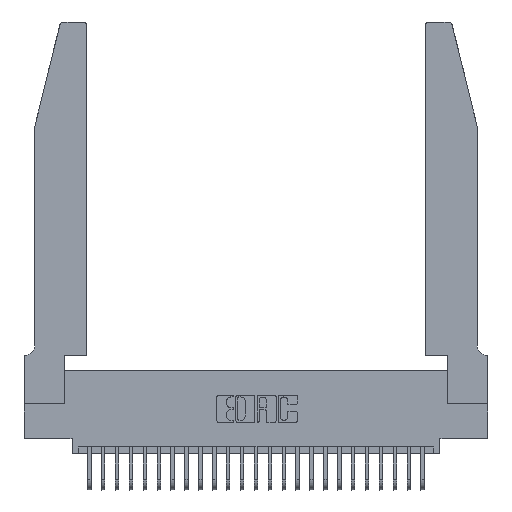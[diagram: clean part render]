
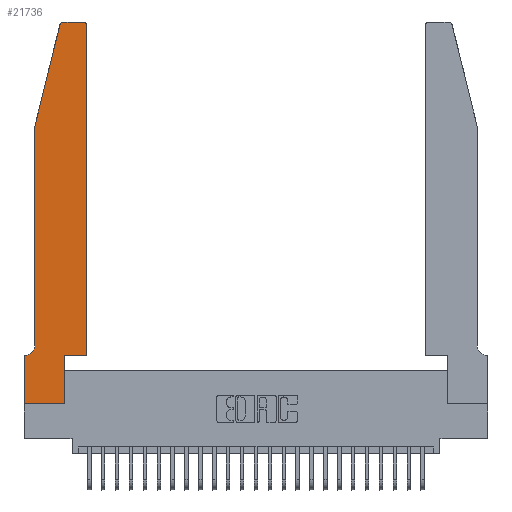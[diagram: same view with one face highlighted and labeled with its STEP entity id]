
A CAD part, top view. The second image highlights one B-rep face of the part: STEP entity #21736.
In plain terms, the highlighted planar face has unit normal (0, 0, 1).
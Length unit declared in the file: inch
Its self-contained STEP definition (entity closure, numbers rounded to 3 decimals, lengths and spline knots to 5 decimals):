
#370 = DIRECTION ( 'NONE',  ( -0.239, -0.971, 0. ) ) ;
#458 = LINE ( 'NONE', #26367, #18158 ) ;
#739 = CARTESIAN_POINT ( 'NONE',  ( 0.0755, 2., 0.37 ) ) ;
#792 = VERTEX_POINT ( 'NONE', #2043 ) ;
#999 = DIRECTION ( 'NONE',  ( 1., 0., 0. ) ) ;
#1038 = EDGE_CURVE ( 'NONE', #14653, #17005, #2026, .T. ) ;
#2026 = LINE ( 'NONE', #13198, #24736 ) ;
#2043 = CARTESIAN_POINT ( 'NONE',  ( 0.25487, 2.72718, 0.37 ) ) ;
#2344 = LINE ( 'NONE', #26648, #13473 ) ;
#2377 = CIRCLE ( 'NONE', #4136, 0.03 ) ;
#2674 = CARTESIAN_POINT ( 'NONE',  ( 0.4205, 2.72, 0.37 ) ) ;
#3915 = CARTESIAN_POINT ( 'NONE',  ( 0.0055, 0.42, 0.37 ) ) ;
#3991 = DIRECTION ( 'NONE',  ( 1., 0., 0. ) ) ;
#4113 = VECTOR ( 'NONE', #16092, 39.37008 ) ;
#4121 = VERTEX_POINT ( 'NONE', #28270 ) ;
#4136 = AXIS2_PLACEMENT_3D ( 'NONE', #2674, #18172, #4959 ) ;
#4201 = LINE ( 'NONE', #13701, #16003 ) ;
#4290 = CARTESIAN_POINT ( 'NONE',  ( 0.284, 2.72, 0.37 ) ) ;
#4513 = LINE ( 'NONE', #6913, #21312 ) ;
#4536 = VERTEX_POINT ( 'NONE', #14696 ) ;
#4736 = EDGE_CURVE ( 'NONE', #6855, #4121, #458, .T. ) ;
#4761 = ORIENTED_EDGE ( 'NONE', *, *, #24069, .T. ) ;
#4855 = ORIENTED_EDGE ( 'NONE', *, *, #20783, .T. ) ;
#4959 = DIRECTION ( 'NONE',  ( 1., 0., 0. ) ) ;
#5266 = LINE ( 'NONE', #25333, #16341 ) ;
#5336 = VERTEX_POINT ( 'NONE', #19955 ) ;
#5622 = VECTOR ( 'NONE', #11057, 39.37008 ) ;
#5817 = CARTESIAN_POINT ( 'NONE',  ( 0.2865, 0., 0.37 ) ) ;
#6170 = DIRECTION ( 'NONE',  ( -1., 0., 0. ) ) ;
#6537 = DIRECTION ( 'NONE',  ( 1., 0., 0. ) ) ;
#6746 = VERTEX_POINT ( 'NONE', #7605 ) ;
#6763 = VERTEX_POINT ( 'NONE', #16480 ) ;
#6855 = VERTEX_POINT ( 'NONE', #21061 ) ;
#6913 = CARTESIAN_POINT ( 'NONE',  ( 0.4505, 0.35, 0.37 ) ) ;
#6969 = DIRECTION ( 'NONE',  ( 0., 1., 0. ) ) ;
#7067 = CARTESIAN_POINT ( 'NONE',  ( 0.4205, 2.75, 0.37 ) ) ;
#7605 = CARTESIAN_POINT ( 'NONE',  ( 0.4505, 2.72, 0.37 ) ) ;
#7697 = CARTESIAN_POINT ( 'NONE',  ( 0., 0.35, 0.37 ) ) ;
#7717 = VERTEX_POINT ( 'NONE', #7067 ) ;
#7966 = LINE ( 'NONE', #26857, #4113 ) ;
#8982 = EDGE_CURVE ( 'NONE', #6763, #792, #11916, .T. ) ;
#9638 = EDGE_CURVE ( 'NONE', #7717, #6763, #17377, .T. ) ;
#10096 = EDGE_CURVE ( 'NONE', #22844, #6855, #12187, .T. ) ;
#10583 = ORIENTED_EDGE ( 'NONE', *, *, #1038, .T. ) ;
#10942 = EDGE_CURVE ( 'NONE', #5336, #6746, #4513, .T. ) ;
#11019 = EDGE_CURVE ( 'NONE', #6746, #7717, #2377, .T. ) ;
#11057 = DIRECTION ( 'NONE',  ( -1., 0., 0. ) ) ;
#11712 = EDGE_CURVE ( 'NONE', #4536, #5336, #7966, .T. ) ;
#11761 = AXIS2_PLACEMENT_3D ( 'NONE', #3915, #19330, #6170 ) ;
#11916 = CIRCLE ( 'NONE', #24123, 0.03 ) ;
#12187 = CIRCLE ( 'NONE', #11761, 0.07 ) ;
#12726 = CARTESIAN_POINT ( 'NONE',  ( 0.0755, 0.42, 0.37 ) ) ;
#13100 = CARTESIAN_POINT ( 'NONE',  ( 0., 0., 0.37 ) ) ;
#13198 = CARTESIAN_POINT ( 'NONE',  ( 0., 0., 0.37 ) ) ;
#13473 = VECTOR ( 'NONE', #6969, 39.37008 ) ;
#13474 = DIRECTION ( 'NONE',  ( 0., 1., 0. ) ) ;
#13701 = CARTESIAN_POINT ( 'NONE',  ( 0.0755, 2., 0.37 ) ) ;
#14337 = DIRECTION ( 'NONE',  ( 0., 0., 1. ) ) ;
#14653 = VERTEX_POINT ( 'NONE', #13100 ) ;
#14696 = CARTESIAN_POINT ( 'NONE',  ( 0.2865, 0.35, 0.37 ) ) ;
#14773 = ORIENTED_EDGE ( 'NONE', *, *, #10942, .T. ) ;
#15584 = DIRECTION ( 'NONE',  ( -1., 0., 0. ) ) ;
#16003 = VECTOR ( 'NONE', #370, 39.37008 ) ;
#16092 = DIRECTION ( 'NONE',  ( 1., 0., 0. ) ) ;
#16341 = VECTOR ( 'NONE', #27480, 39.37008 ) ;
#16480 = CARTESIAN_POINT ( 'NONE',  ( 0.284, 2.75, 0.37 ) ) ;
#16810 = VECTOR ( 'NONE', #26281, 39.37008 ) ;
#17005 = VERTEX_POINT ( 'NONE', #5817 ) ;
#17377 = LINE ( 'NONE', #24086, #5622 ) ;
#18158 = VECTOR ( 'NONE', #15584, 39.37008 ) ;
#18172 = DIRECTION ( 'NONE',  ( 0., 0., 1. ) ) ;
#18175 = EDGE_CURVE ( 'NONE', #17005, #4536, #2344, .T. ) ;
#18342 = AXIS2_PLACEMENT_3D ( 'NONE', #7697, #14337, #999 ) ;
#18561 = ORIENTED_EDGE ( 'NONE', *, *, #11019, .T. ) ;
#19330 = DIRECTION ( 'NONE',  ( 0., 0., -1. ) ) ;
#19687 = DIRECTION ( 'NONE',  ( 0., 0., 1. ) ) ;
#19955 = CARTESIAN_POINT ( 'NONE',  ( 0.4505, 0.35, 0.37 ) ) ;
#20783 = EDGE_CURVE ( 'NONE', #27594, #22844, #28310, .T. ) ;
#21061 = CARTESIAN_POINT ( 'NONE',  ( 0.0055, 0.35, 0.37 ) ) ;
#21090 = ORIENTED_EDGE ( 'NONE', *, *, #8982, .T. ) ;
#21312 = VECTOR ( 'NONE', #13474, 39.37008 ) ;
#21483 = ORIENTED_EDGE ( 'NONE', *, *, #24328, .T. ) ;
#21736 = ADVANCED_FACE ( 'NONE', ( #21782 ), #25083, .T. ) ;
#21782 = FACE_OUTER_BOUND ( 'NONE', #26757, .T. ) ;
#22844 = VERTEX_POINT ( 'NONE', #12726 ) ;
#23301 = ORIENTED_EDGE ( 'NONE', *, *, #4736, .T. ) ;
#23458 = ORIENTED_EDGE ( 'NONE', *, *, #18175, .T. ) ;
#24062 = CARTESIAN_POINT ( 'NONE',  ( 0.0755, 2., 0.37 ) ) ;
#24069 = EDGE_CURVE ( 'NONE', #4121, #14653, #5266, .T. ) ;
#24086 = CARTESIAN_POINT ( 'NONE',  ( 0.2605, 2.75, 0.37 ) ) ;
#24123 = AXIS2_PLACEMENT_3D ( 'NONE', #4290, #19687, #6537 ) ;
#24328 = EDGE_CURVE ( 'NONE', #792, #27594, #4201, .T. ) ;
#24736 = VECTOR ( 'NONE', #3991, 39.37008 ) ;
#25083 = PLANE ( 'NONE',  #18342 ) ;
#25333 = CARTESIAN_POINT ( 'NONE',  ( 0., 0., 0.37 ) ) ;
#25919 = ORIENTED_EDGE ( 'NONE', *, *, #11712, .T. ) ;
#26281 = DIRECTION ( 'NONE',  ( 0., -1., 0. ) ) ;
#26367 = CARTESIAN_POINT ( 'NONE',  ( 0.0755, 0.35, 0.37 ) ) ;
#26648 = CARTESIAN_POINT ( 'NONE',  ( 0.2865, 0.35, 0.37 ) ) ;
#26757 = EDGE_LOOP ( 'NONE', ( #27772, #21090, #21483, #4855, #26826, #23301, #4761, #10583, #23458, #25919, #14773, #18561 ) ) ;
#26826 = ORIENTED_EDGE ( 'NONE', *, *, #10096, .T. ) ;
#26857 = CARTESIAN_POINT ( 'NONE',  ( 0.4505, 0.35, 0.37 ) ) ;
#27480 = DIRECTION ( 'NONE',  ( 0., -1., 0. ) ) ;
#27594 = VERTEX_POINT ( 'NONE', #739 ) ;
#27772 = ORIENTED_EDGE ( 'NONE', *, *, #9638, .T. ) ;
#28270 = CARTESIAN_POINT ( 'NONE',  ( 0., 0.35, 0.37 ) ) ;
#28310 = LINE ( 'NONE', #24062, #16810 ) ;
